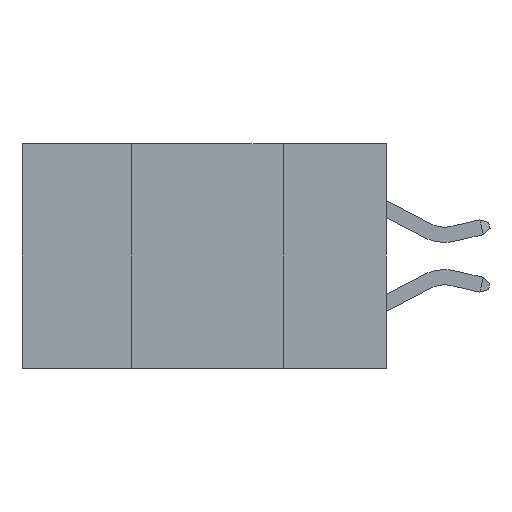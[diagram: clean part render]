
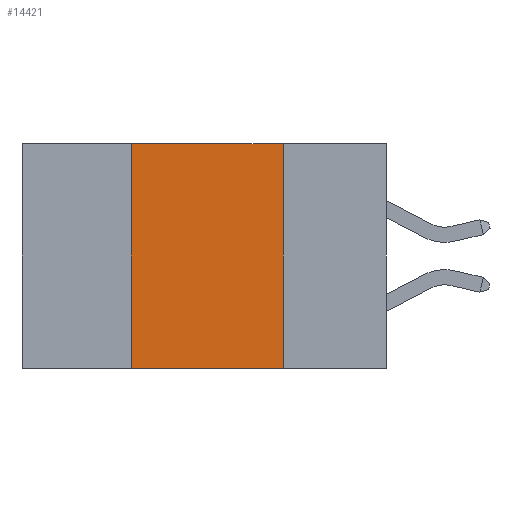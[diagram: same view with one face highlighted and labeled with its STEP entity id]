
A CAD part, left-side view. The second image highlights one B-rep face of the part: STEP entity #14421.
In plain terms, the highlighted planar face has unit normal (-1, 0, 0).
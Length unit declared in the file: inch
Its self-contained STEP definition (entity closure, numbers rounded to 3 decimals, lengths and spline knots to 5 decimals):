
#152 = CARTESIAN_POINT ( 'NONE',  ( 0., 0.17, 0. ) ) ;
#641 = LINE ( 'NONE', #3815, #4236 ) ;
#816 = DIRECTION ( 'NONE',  ( 0., 0., 1. ) ) ;
#1165 = VECTOR ( 'NONE', #2988, 39.37008 ) ;
#1854 = PLANE ( 'NONE',  #7961 ) ;
#1936 = ORIENTED_EDGE ( 'NONE', *, *, #8939, .F. ) ;
#2831 = EDGE_CURVE ( 'NONE', #3781, #18522, #18923, .T. ) ;
#2911 = CARTESIAN_POINT ( 'NONE',  ( 0., 0.6, 0. ) ) ;
#2988 = DIRECTION ( 'NONE',  ( 0., -1., 0. ) ) ;
#3781 = VERTEX_POINT ( 'NONE', #8286 ) ;
#3815 = CARTESIAN_POINT ( 'NONE',  ( 0., 0.42, 0. ) ) ;
#4095 = FACE_OUTER_BOUND ( 'NONE', #16247, .T. ) ;
#4236 = VECTOR ( 'NONE', #816, 39.37008 ) ;
#4557 = CARTESIAN_POINT ( 'NONE',  ( 0., 0.6, -0.37 ) ) ;
#4952 = DIRECTION ( 'NONE',  ( 1., 0., 0. ) ) ;
#5905 = EDGE_CURVE ( 'NONE', #15565, #18522, #16323, .T. ) ;
#6065 = DIRECTION ( 'NONE',  ( 0., -1., 0. ) ) ;
#7185 = DIRECTION ( 'NONE',  ( 0., 0., -1. ) ) ;
#7258 = ORIENTED_EDGE ( 'NONE', *, *, #2831, .F. ) ;
#7652 = CARTESIAN_POINT ( 'NONE',  ( 0., 0.17, -0.37 ) ) ;
#7961 = AXIS2_PLACEMENT_3D ( 'NONE', #15373, #4952, #15435 ) ;
#8019 = EDGE_CURVE ( 'NONE', #13389, #3781, #9228, .T. ) ;
#8286 = CARTESIAN_POINT ( 'NONE',  ( 0., 0.17, 0. ) ) ;
#8939 = EDGE_CURVE ( 'NONE', #15565, #13389, #641, .T. ) ;
#9228 = LINE ( 'NONE', #2911, #1165 ) ;
#11112 = VECTOR ( 'NONE', #7185, 39.37008 ) ;
#11446 = VECTOR ( 'NONE', #6065, 39.37008 ) ;
#13389 = VERTEX_POINT ( 'NONE', #18726 ) ;
#13535 = ORIENTED_EDGE ( 'NONE', *, *, #8019, .F. ) ;
#14421 = ADVANCED_FACE ( 'NONE', ( #4095 ), #1854, .F. ) ;
#15373 = CARTESIAN_POINT ( 'NONE',  ( 0., 0.6, 0. ) ) ;
#15435 = DIRECTION ( 'NONE',  ( 0., 0., -1. ) ) ;
#15565 = VERTEX_POINT ( 'NONE', #16598 ) ;
#15721 = ORIENTED_EDGE ( 'NONE', *, *, #5905, .T. ) ;
#16247 = EDGE_LOOP ( 'NONE', ( #7258, #13535, #1936, #15721 ) ) ;
#16323 = LINE ( 'NONE', #4557, #11446 ) ;
#16598 = CARTESIAN_POINT ( 'NONE',  ( 0., 0.42, -0.37 ) ) ;
#18522 = VERTEX_POINT ( 'NONE', #7652 ) ;
#18726 = CARTESIAN_POINT ( 'NONE',  ( 0., 0.42, 0. ) ) ;
#18923 = LINE ( 'NONE', #152, #11112 ) ;
